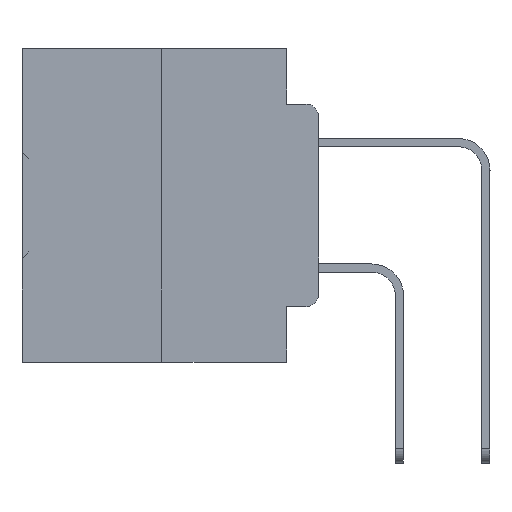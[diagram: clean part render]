
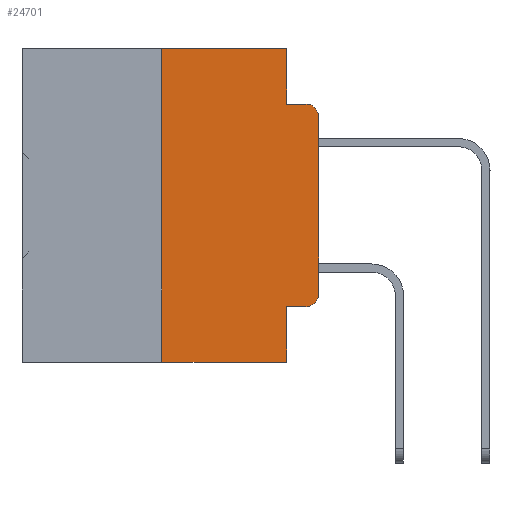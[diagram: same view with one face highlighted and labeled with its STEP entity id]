
A CAD part, left-side view. The second image highlights one B-rep face of the part: STEP entity #24701.
In plain terms, the highlighted planar face has unit normal (-1, 0, 0).
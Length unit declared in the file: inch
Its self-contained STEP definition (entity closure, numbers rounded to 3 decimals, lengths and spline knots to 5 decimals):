
#197 = AXIS2_PLACEMENT_3D ( 'NONE', #4293, #7348, #25706 ) ;
#300 = CARTESIAN_POINT ( 'NONE',  ( 0., 0.02, -0.0885 ) ) ;
#431 = ORIENTED_EDGE ( 'NONE', *, *, #31354, .T. ) ;
#584 = VECTOR ( 'NONE', #2124, 39.37008 ) ;
#615 = CARTESIAN_POINT ( 'NONE',  ( 0., 0.25, 0. ) ) ;
#622 = CARTESIAN_POINT ( 'NONE',  ( 0., 0.473, 0. ) ) ;
#846 = VECTOR ( 'NONE', #27551, 39.37008 ) ;
#879 = VERTEX_POINT ( 'NONE', #23003 ) ;
#1099 = VERTEX_POINT ( 'NONE', #13859 ) ;
#1117 = EDGE_CURVE ( 'NONE', #7189, #1099, #32839, .T. ) ;
#2124 = DIRECTION ( 'NONE',  ( 0., -1., 0. ) ) ;
#2522 = CARTESIAN_POINT ( 'NONE',  ( 0., 0.25, 0. ) ) ;
#4293 = CARTESIAN_POINT ( 'NONE',  ( 0., 0.02, -0.1085 ) ) ;
#5823 = DIRECTION ( 'NONE',  ( 0., 0., -1. ) ) ;
#6743 = LINE ( 'NONE', #2522, #15826 ) ;
#6926 = VERTEX_POINT ( 'NONE', #615 ) ;
#7189 = VERTEX_POINT ( 'NONE', #24439 ) ;
#7348 = DIRECTION ( 'NONE',  ( -1., 0., 0. ) ) ;
#7421 = CARTESIAN_POINT ( 'NONE',  ( 0., 0.25, -0.5 ) ) ;
#7688 = LINE ( 'NONE', #17614, #584 ) ;
#7989 = CARTESIAN_POINT ( 'NONE',  ( 0., 0.02, -0.3915 ) ) ;
#8050 = CARTESIAN_POINT ( 'NONE',  ( 0., 0.051, 0. ) ) ;
#8718 = VERTEX_POINT ( 'NONE', #27891 ) ;
#9138 = CARTESIAN_POINT ( 'NONE',  ( 0., 0.051, 0. ) ) ;
#9997 = VERTEX_POINT ( 'NONE', #13736 ) ;
#10377 = ORIENTED_EDGE ( 'NONE', *, *, #20516, .F. ) ;
#10549 = VECTOR ( 'NONE', #18208, 39.37008 ) ;
#11072 = DIRECTION ( 'NONE',  ( 0., 0., -1. ) ) ;
#11887 = VERTEX_POINT ( 'NONE', #7421 ) ;
#12156 = CARTESIAN_POINT ( 'NONE',  ( 0., 0.051, 0. ) ) ;
#13228 = ORIENTED_EDGE ( 'NONE', *, *, #18394, .F. ) ;
#13428 = ORIENTED_EDGE ( 'NONE', *, *, #1117, .T. ) ;
#13736 = CARTESIAN_POINT ( 'NONE',  ( 0., 0.051, -0.4115 ) ) ;
#13859 = CARTESIAN_POINT ( 'NONE',  ( 0., 0., -0.1085 ) ) ;
#13890 = VERTEX_POINT ( 'NONE', #8050 ) ;
#15826 = VECTOR ( 'NONE', #30023, 39.37008 ) ;
#16050 = PLANE ( 'NONE',  #24355 ) ;
#17614 = CARTESIAN_POINT ( 'NONE',  ( 0., 0.473, -0.5 ) ) ;
#18208 = DIRECTION ( 'NONE',  ( 0., -1., 0. ) ) ;
#18394 = EDGE_CURVE ( 'NONE', #879, #21470, #33210, .T. ) ;
#18685 = FACE_OUTER_BOUND ( 'NONE', #31312, .T. ) ;
#19435 = DIRECTION ( 'NONE',  ( 0., -1., 0. ) ) ;
#19794 = ORIENTED_EDGE ( 'NONE', *, *, #38541, .T. ) ;
#19874 = EDGE_CURVE ( 'NONE', #13890, #879, #37194, .T. ) ;
#20339 = ORIENTED_EDGE ( 'NONE', *, *, #27411, .F. ) ;
#20516 = EDGE_CURVE ( 'NONE', #9997, #27938, #33325, .T. ) ;
#20873 = CIRCLE ( 'NONE', #197, 0.02 ) ;
#21012 = ORIENTED_EDGE ( 'NONE', *, *, #26625, .F. ) ;
#21470 = VERTEX_POINT ( 'NONE', #300 ) ;
#21823 = CARTESIAN_POINT ( 'NONE',  ( 0., 0.051, -0.4115 ) ) ;
#23003 = CARTESIAN_POINT ( 'NONE',  ( 0., 0.051, -0.0885 ) ) ;
#24248 = VECTOR ( 'NONE', #29798, 39.37008 ) ;
#24355 = AXIS2_PLACEMENT_3D ( 'NONE', #31158, #37459, #25323 ) ;
#24439 = CARTESIAN_POINT ( 'NONE',  ( 0., 0., -0.3915 ) ) ;
#24701 = ADVANCED_FACE ( 'NONE', ( #18685 ), #16050, .F. ) ;
#25323 = DIRECTION ( 'NONE',  ( 0., 0., -1. ) ) ;
#25706 = DIRECTION ( 'NONE',  ( 0., 0., -1. ) ) ;
#26472 = LINE ( 'NONE', #622, #29817 ) ;
#26625 = EDGE_CURVE ( 'NONE', #6926, #13890, #26472, .T. ) ;
#27348 = AXIS2_PLACEMENT_3D ( 'NONE', #7989, #29383, #11072 ) ;
#27391 = CIRCLE ( 'NONE', #27348, 0.02 ) ;
#27411 = EDGE_CURVE ( 'NONE', #11887, #6926, #6743, .T. ) ;
#27551 = DIRECTION ( 'NONE',  ( 0., 0., -1. ) ) ;
#27891 = CARTESIAN_POINT ( 'NONE',  ( 0., 0.02, -0.4115 ) ) ;
#27938 = VERTEX_POINT ( 'NONE', #32533 ) ;
#28355 = DIRECTION ( 'NONE',  ( 0., -1., 0. ) ) ;
#28570 = ORIENTED_EDGE ( 'NONE', *, *, #36836, .T. ) ;
#29383 = DIRECTION ( 'NONE',  ( -1., 0., 0. ) ) ;
#29798 = DIRECTION ( 'NONE',  ( 0., 0., 1. ) ) ;
#29817 = VECTOR ( 'NONE', #28355, 39.37008 ) ;
#30023 = DIRECTION ( 'NONE',  ( 0., 0., 1. ) ) ;
#31158 = CARTESIAN_POINT ( 'NONE',  ( 0., 0.473, 0. ) ) ;
#31312 = EDGE_LOOP ( 'NONE', ( #13428, #431, #13228, #38651, #21012, #20339, #28570, #10377, #31632, #19794 ) ) ;
#31354 = EDGE_CURVE ( 'NONE', #1099, #21470, #20873, .T. ) ;
#31632 = ORIENTED_EDGE ( 'NONE', *, *, #39142, .T. ) ;
#32533 = CARTESIAN_POINT ( 'NONE',  ( 0., 0.051, -0.5 ) ) ;
#32839 = LINE ( 'NONE', #35813, #24248 ) ;
#33210 = LINE ( 'NONE', #37712, #35119 ) ;
#33325 = LINE ( 'NONE', #12156, #846 ) ;
#35119 = VECTOR ( 'NONE', #19435, 39.37008 ) ;
#35813 = CARTESIAN_POINT ( 'NONE',  ( 0., 0., 0. ) ) ;
#36836 = EDGE_CURVE ( 'NONE', #11887, #27938, #7688, .T. ) ;
#36897 = LINE ( 'NONE', #21823, #10549 ) ;
#37194 = LINE ( 'NONE', #9138, #37672 ) ;
#37459 = DIRECTION ( 'NONE',  ( 1., 0., 0. ) ) ;
#37672 = VECTOR ( 'NONE', #5823, 39.37008 ) ;
#37712 = CARTESIAN_POINT ( 'NONE',  ( 0., 0.051, -0.0885 ) ) ;
#38541 = EDGE_CURVE ( 'NONE', #8718, #7189, #27391, .T. ) ;
#38651 = ORIENTED_EDGE ( 'NONE', *, *, #19874, .F. ) ;
#39142 = EDGE_CURVE ( 'NONE', #9997, #8718, #36897, .T. ) ;
